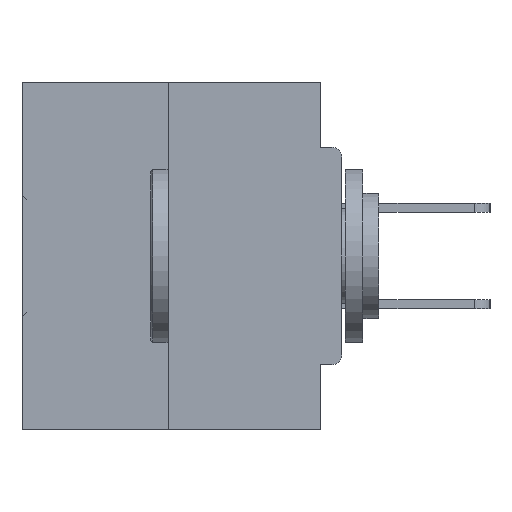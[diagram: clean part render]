
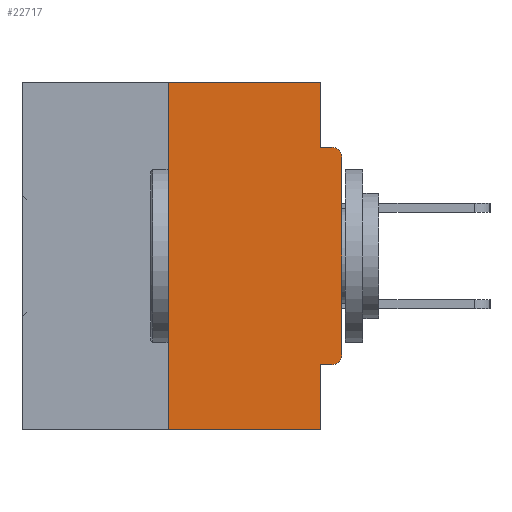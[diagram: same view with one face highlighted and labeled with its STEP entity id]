
A CAD part, left-side view. The second image highlights one B-rep face of the part: STEP entity #22717.
In plain terms, the highlighted planar face has unit normal (-1, 0, 0).
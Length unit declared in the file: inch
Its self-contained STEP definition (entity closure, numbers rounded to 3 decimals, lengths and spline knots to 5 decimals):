
#569 = CARTESIAN_POINT ( 'NONE',  ( 0., 0.015, -0.3915 ) ) ;
#706 = VECTOR ( 'NONE', #1579, 39.37008 ) ;
#1579 = DIRECTION ( 'NONE',  ( 0., 0., 1. ) ) ;
#1762 = LINE ( 'NONE', #34342, #28630 ) ;
#3213 = EDGE_CURVE ( 'NONE', #33499, #5414, #15540, .T. ) ;
#3597 = ORIENTED_EDGE ( 'NONE', *, *, #38611, .T. ) ;
#3609 = EDGE_CURVE ( 'NONE', #5414, #16423, #39604, .T. ) ;
#4634 = CARTESIAN_POINT ( 'NONE',  ( 0., 0., -0.4065 ) ) ;
#5041 = DIRECTION ( 'NONE',  ( 0., 0., 1. ) ) ;
#5181 = EDGE_CURVE ( 'NONE', #22258, #24179, #23523, .T. ) ;
#5285 = AXIS2_PLACEMENT_3D ( 'NONE', #26992, #5994, #9647 ) ;
#5414 = VERTEX_POINT ( 'NONE', #10730 ) ;
#5531 = FACE_OUTER_BOUND ( 'NONE', #8210, .T. ) ;
#5994 = DIRECTION ( 'NONE',  ( -1., 0., 0. ) ) ;
#6144 = ORIENTED_EDGE ( 'NONE', *, *, #41780, .T. ) ;
#6201 = ORIENTED_EDGE ( 'NONE', *, *, #8793, .F. ) ;
#6496 = VECTOR ( 'NONE', #11704, 39.37008 ) ;
#7214 = EDGE_CURVE ( 'NONE', #30851, #34003, #15186, .T. ) ;
#7228 = DIRECTION ( 'NONE',  ( 0., -1., 0. ) ) ;
#8210 = EDGE_LOOP ( 'NONE', ( #6201, #34515, #3597, #15934, #30425, #10931, #6144, #29007, #34846, #16930 ) ) ;
#8385 = VECTOR ( 'NONE', #23600, 39.37008 ) ;
#8793 = EDGE_CURVE ( 'NONE', #24179, #36887, #40586, .T. ) ;
#9647 = DIRECTION ( 'NONE',  ( 0., 0., -1. ) ) ;
#10306 = AXIS2_PLACEMENT_3D ( 'NONE', #569, #14497, #18042 ) ;
#10597 = VECTOR ( 'NONE', #39854, 39.37008 ) ;
#10730 = CARTESIAN_POINT ( 'NONE',  ( 0., 0.031, -0.4065 ) ) ;
#10931 = ORIENTED_EDGE ( 'NONE', *, *, #31820, .T. ) ;
#11202 = DIRECTION ( 'NONE',  ( 1., 0., 0. ) ) ;
#11247 = CIRCLE ( 'NONE', #10306, 0.015 ) ;
#11668 = CARTESIAN_POINT ( 'NONE',  ( 0., 0.031, -0.5 ) ) ;
#11704 = DIRECTION ( 'NONE',  ( 0., -1., 0. ) ) ;
#12491 = CARTESIAN_POINT ( 'NONE',  ( 0., 0.25, 0. ) ) ;
#13470 = DIRECTION ( 'NONE',  ( 0., 0., -1. ) ) ;
#14240 = VECTOR ( 'NONE', #25914, 39.37008 ) ;
#14497 = DIRECTION ( 'NONE',  ( -1., 0., 0. ) ) ;
#14737 = DIRECTION ( 'NONE',  ( 0., 0., -1. ) ) ;
#15186 = CIRCLE ( 'NONE', #5285, 0.015 ) ;
#15540 = LINE ( 'NONE', #4634, #10597 ) ;
#15934 = ORIENTED_EDGE ( 'NONE', *, *, #3609, .F. ) ;
#16423 = VERTEX_POINT ( 'NONE', #25761 ) ;
#16930 = ORIENTED_EDGE ( 'NONE', *, *, #33761, .F. ) ;
#18014 = CARTESIAN_POINT ( 'NONE',  ( 0., 0.25, 0. ) ) ;
#18042 = DIRECTION ( 'NONE',  ( 0., 0., -1. ) ) ;
#18416 = CARTESIAN_POINT ( 'NONE',  ( 0., 0.46, 0. ) ) ;
#20996 = AXIS2_PLACEMENT_3D ( 'NONE', #43094, #11202, #14737 ) ;
#21077 = CARTESIAN_POINT ( 'NONE',  ( 0., 0.031, 0. ) ) ;
#21338 = VECTOR ( 'NONE', #7228, 39.37008 ) ;
#21555 = LINE ( 'NONE', #36520, #706 ) ;
#21704 = CARTESIAN_POINT ( 'NONE',  ( 0., 0.25, -0.5 ) ) ;
#22167 = CARTESIAN_POINT ( 'NONE',  ( 0., 0., -0.0935 ) ) ;
#22258 = VERTEX_POINT ( 'NONE', #21704 ) ;
#22562 = CARTESIAN_POINT ( 'NONE',  ( 0., 0.031, -0.0935 ) ) ;
#22717 = ADVANCED_FACE ( 'NONE', ( #5531 ), #42476, .F. ) ;
#23523 = LINE ( 'NONE', #12491, #35613 ) ;
#23600 = DIRECTION ( 'NONE',  ( 0., 0., -1. ) ) ;
#24179 = VERTEX_POINT ( 'NONE', #18014 ) ;
#25761 = CARTESIAN_POINT ( 'NONE',  ( 0., 0.031, -0.5 ) ) ;
#25914 = DIRECTION ( 'NONE',  ( 0., -1., 0. ) ) ;
#26820 = LINE ( 'NONE', #35385, #21338 ) ;
#26992 = CARTESIAN_POINT ( 'NONE',  ( 0., 0.015, -0.1085 ) ) ;
#28630 = VECTOR ( 'NONE', #13470, 39.37008 ) ;
#29007 = ORIENTED_EDGE ( 'NONE', *, *, #7214, .T. ) ;
#29414 = EDGE_CURVE ( 'NONE', #45356, #34003, #37740, .T. ) ;
#29496 = CARTESIAN_POINT ( 'NONE',  ( 0., 0.015, -0.4065 ) ) ;
#30425 = ORIENTED_EDGE ( 'NONE', *, *, #3213, .F. ) ;
#30851 = VERTEX_POINT ( 'NONE', #37188 ) ;
#31820 = EDGE_CURVE ( 'NONE', #33499, #40075, #11247, .T. ) ;
#33109 = CARTESIAN_POINT ( 'NONE',  ( 0., 0.015, -0.0935 ) ) ;
#33499 = VERTEX_POINT ( 'NONE', #29496 ) ;
#33761 = EDGE_CURVE ( 'NONE', #36887, #45356, #1762, .T. ) ;
#34003 = VERTEX_POINT ( 'NONE', #33109 ) ;
#34342 = CARTESIAN_POINT ( 'NONE',  ( 0., 0.031, 0. ) ) ;
#34515 = ORIENTED_EDGE ( 'NONE', *, *, #5181, .F. ) ;
#34846 = ORIENTED_EDGE ( 'NONE', *, *, #29414, .F. ) ;
#35321 = CARTESIAN_POINT ( 'NONE',  ( 0., 0., -0.3915 ) ) ;
#35385 = CARTESIAN_POINT ( 'NONE',  ( 0., 0.46, -0.5 ) ) ;
#35613 = VECTOR ( 'NONE', #5041, 39.37008 ) ;
#36520 = CARTESIAN_POINT ( 'NONE',  ( 0., 0., 0. ) ) ;
#36887 = VERTEX_POINT ( 'NONE', #21077 ) ;
#37188 = CARTESIAN_POINT ( 'NONE',  ( 0., 0., -0.1085 ) ) ;
#37740 = LINE ( 'NONE', #22167, #6496 ) ;
#38611 = EDGE_CURVE ( 'NONE', #22258, #16423, #26820, .T. ) ;
#39604 = LINE ( 'NONE', #11668, #8385 ) ;
#39854 = DIRECTION ( 'NONE',  ( 0., 1., 0. ) ) ;
#40075 = VERTEX_POINT ( 'NONE', #35321 ) ;
#40586 = LINE ( 'NONE', #18416, #14240 ) ;
#41780 = EDGE_CURVE ( 'NONE', #40075, #30851, #21555, .T. ) ;
#42476 = PLANE ( 'NONE',  #20996 ) ;
#43094 = CARTESIAN_POINT ( 'NONE',  ( 0., 0.46, 0. ) ) ;
#45356 = VERTEX_POINT ( 'NONE', #22562 ) ;
